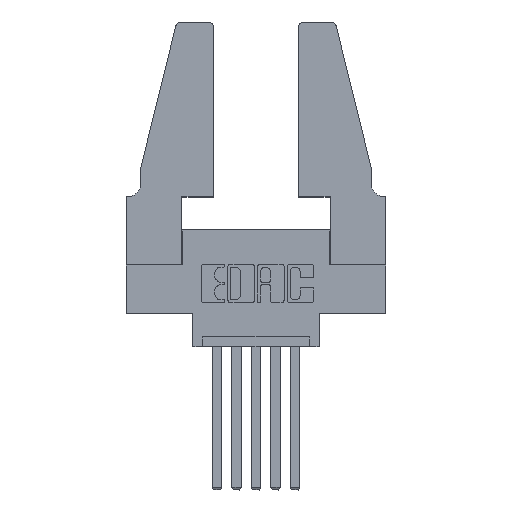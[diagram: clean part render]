
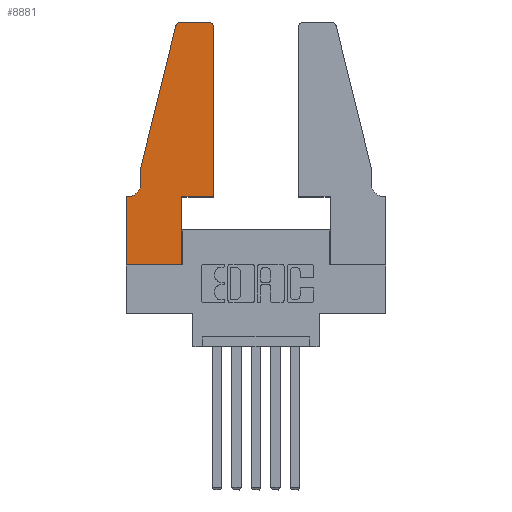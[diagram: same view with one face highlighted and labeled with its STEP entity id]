
A CAD part, top view. The second image highlights one B-rep face of the part: STEP entity #8881.
In plain terms, the highlighted planar face has unit normal (0, 0, 1).
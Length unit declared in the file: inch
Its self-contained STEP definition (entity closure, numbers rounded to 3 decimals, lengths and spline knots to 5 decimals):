
#51 = ORIENTED_EDGE ( 'NONE', *, *, #616, .T. ) ;
#91 = LINE ( 'NONE', #6774, #6468 ) ;
#209 = DIRECTION ( 'NONE',  ( 0., 0., 1. ) ) ;
#402 = AXIS2_PLACEMENT_3D ( 'NONE', #3626, #8668, #4568 ) ;
#415 = VERTEX_POINT ( 'NONE', #6234 ) ;
#616 = EDGE_CURVE ( 'NONE', #1237, #3128, #10781, .T. ) ;
#669 = ORIENTED_EDGE ( 'NONE', *, *, #1518, .T. ) ;
#771 = AXIS2_PLACEMENT_3D ( 'NONE', #8597, #209, #8660 ) ;
#1116 = ORIENTED_EDGE ( 'NONE', *, *, #4676, .T. ) ;
#1237 = VERTEX_POINT ( 'NONE', #10188 ) ;
#1250 = ORIENTED_EDGE ( 'NONE', *, *, #7082, .T. ) ;
#1518 = EDGE_CURVE ( 'NONE', #6402, #9654, #10625, .T. ) ;
#1603 = EDGE_CURVE ( 'NONE', #9789, #9514, #8399, .T. ) ;
#1641 = DIRECTION ( 'NONE',  ( 0., -1., 0. ) ) ;
#1747 = VECTOR ( 'NONE', #6673, 39.37008 ) ;
#1919 = PLANE ( 'NONE',  #771 ) ;
#2002 = LINE ( 'NONE', #3470, #1747 ) ;
#2590 = DIRECTION ( 'NONE',  ( 0., -1., 0. ) ) ;
#2674 = VERTEX_POINT ( 'NONE', #9841 ) ;
#2736 = CARTESIAN_POINT ( 'NONE',  ( 0., 0., 0.37 ) ) ;
#2806 = CARTESIAN_POINT ( 'NONE',  ( 0.0755, 0.42, 0.37 ) ) ;
#3128 = VERTEX_POINT ( 'NONE', #8133 ) ;
#3470 = CARTESIAN_POINT ( 'NONE',  ( 0.0755, 0.35, 0.37 ) ) ;
#3584 = DIRECTION ( 'NONE',  ( 1., 0., 0. ) ) ;
#3597 = CIRCLE ( 'NONE', #9255, 0.03 ) ;
#3626 = CARTESIAN_POINT ( 'NONE',  ( 0.0055, 0.42, 0.37 ) ) ;
#3688 = CARTESIAN_POINT ( 'NONE',  ( 0., 0.35, 0.37 ) ) ;
#3951 = DIRECTION ( 'NONE',  ( 0., 1., 0. ) ) ;
#4238 = CIRCLE ( 'NONE', #402, 0.07 ) ;
#4302 = EDGE_CURVE ( 'NONE', #9654, #9288, #3597, .T. ) ;
#4568 = DIRECTION ( 'NONE',  ( -1., 0., 0. ) ) ;
#4573 = DIRECTION ( 'NONE',  ( 1., 0., 0. ) ) ;
#4646 = LINE ( 'NONE', #8347, #8072 ) ;
#4676 = EDGE_CURVE ( 'NONE', #9514, #6031, #4238, .T. ) ;
#4728 = CARTESIAN_POINT ( 'NONE',  ( 0.2605, 1.25, 0.37 ) ) ;
#4741 = ORIENTED_EDGE ( 'NONE', *, *, #1603, .T. ) ;
#5018 = VERTEX_POINT ( 'NONE', #6386 ) ;
#5181 = ORIENTED_EDGE ( 'NONE', *, *, #5581, .T. ) ;
#5260 = LINE ( 'NONE', #2736, #5277 ) ;
#5277 = VECTOR ( 'NONE', #3584, 39.37008 ) ;
#5581 = EDGE_CURVE ( 'NONE', #2674, #1237, #8578, .T. ) ;
#5606 = CARTESIAN_POINT ( 'NONE',  ( 0.284, 1.22, 0.37 ) ) ;
#5708 = ORIENTED_EDGE ( 'NONE', *, *, #8925, .T. ) ;
#5906 = CARTESIAN_POINT ( 'NONE',  ( 0.25487, 1.22718, 0.37 ) ) ;
#6031 = VERTEX_POINT ( 'NONE', #8395 ) ;
#6033 = VECTOR ( 'NONE', #9230, 39.37008 ) ;
#6234 = CARTESIAN_POINT ( 'NONE',  ( 0., 0., 0.37 ) ) ;
#6386 = CARTESIAN_POINT ( 'NONE',  ( 0.2865, 0., 0.37 ) ) ;
#6402 = VERTEX_POINT ( 'NONE', #8605 ) ;
#6468 = VECTOR ( 'NONE', #2590, 39.37008 ) ;
#6477 = CARTESIAN_POINT ( 'NONE',  ( 0.0755, 0.5, 0.37 ) ) ;
#6502 = DIRECTION ( 'NONE',  ( -0.239, -0.971, 0. ) ) ;
#6504 = CARTESIAN_POINT ( 'NONE',  ( 0.4505, 0.35, 0.37 ) ) ;
#6572 = VECTOR ( 'NONE', #9714, 39.37008 ) ;
#6673 = DIRECTION ( 'NONE',  ( -1., 0., 0. ) ) ;
#6753 = ORIENTED_EDGE ( 'NONE', *, *, #9842, .T. ) ;
#6774 = CARTESIAN_POINT ( 'NONE',  ( 0., 0., 0.37 ) ) ;
#6972 = EDGE_CURVE ( 'NONE', #9288, #9789, #4646, .T. ) ;
#6982 = AXIS2_PLACEMENT_3D ( 'NONE', #7189, #9736, #4573 ) ;
#7082 = EDGE_CURVE ( 'NONE', #3128, #6402, #8204, .T. ) ;
#7117 = ORIENTED_EDGE ( 'NONE', *, *, #7146, .T. ) ;
#7146 = EDGE_CURVE ( 'NONE', #9051, #415, #91, .T. ) ;
#7189 = CARTESIAN_POINT ( 'NONE',  ( 0.4205, 1.22, 0.37 ) ) ;
#7245 = DIRECTION ( 'NONE',  ( 0., 0., 1. ) ) ;
#7310 = DIRECTION ( 'NONE',  ( -1., 0., 0. ) ) ;
#7571 = ORIENTED_EDGE ( 'NONE', *, *, #6972, .T. ) ;
#7639 = VECTOR ( 'NONE', #3951, 39.37008 ) ;
#7750 = VECTOR ( 'NONE', #1641, 39.37008 ) ;
#7915 = EDGE_LOOP ( 'NONE', ( #669, #9835, #7571, #4741, #1116, #7928, #7117, #5708, #6753, #5181, #51, #1250 ) ) ;
#7928 = ORIENTED_EDGE ( 'NONE', *, *, #9399, .T. ) ;
#8072 = VECTOR ( 'NONE', #6502, 39.37008 ) ;
#8133 = CARTESIAN_POINT ( 'NONE',  ( 0.4505, 1.22, 0.37 ) ) ;
#8204 = CIRCLE ( 'NONE', #6982, 0.03 ) ;
#8347 = CARTESIAN_POINT ( 'NONE',  ( 0.0755, 0.5, 0.37 ) ) ;
#8395 = CARTESIAN_POINT ( 'NONE',  ( 0.0055, 0.35, 0.37 ) ) ;
#8399 = LINE ( 'NONE', #6477, #7750 ) ;
#8578 = LINE ( 'NONE', #10343, #6572 ) ;
#8597 = CARTESIAN_POINT ( 'NONE',  ( 0., 0.35, 0.37 ) ) ;
#8605 = CARTESIAN_POINT ( 'NONE',  ( 0.4205, 1.25, 0.37 ) ) ;
#8660 = DIRECTION ( 'NONE',  ( 1., 0., 0. ) ) ;
#8668 = DIRECTION ( 'NONE',  ( 0., 0., -1. ) ) ;
#8881 = ADVANCED_FACE ( 'NONE', ( #9493 ), #1919, .T. ) ;
#8925 = EDGE_CURVE ( 'NONE', #415, #5018, #5260, .T. ) ;
#9011 = CARTESIAN_POINT ( 'NONE',  ( 0.0755, 0.5, 0.37 ) ) ;
#9048 = DIRECTION ( 'NONE',  ( 1., 0., 0. ) ) ;
#9051 = VERTEX_POINT ( 'NONE', #3688 ) ;
#9230 = DIRECTION ( 'NONE',  ( 0., 1., 0. ) ) ;
#9255 = AXIS2_PLACEMENT_3D ( 'NONE', #5606, #7245, #9048 ) ;
#9288 = VERTEX_POINT ( 'NONE', #5906 ) ;
#9332 = VECTOR ( 'NONE', #7310, 39.37008 ) ;
#9399 = EDGE_CURVE ( 'NONE', #6031, #9051, #2002, .T. ) ;
#9493 = FACE_OUTER_BOUND ( 'NONE', #7915, .T. ) ;
#9514 = VERTEX_POINT ( 'NONE', #2806 ) ;
#9608 = CARTESIAN_POINT ( 'NONE',  ( 0.284, 1.25, 0.37 ) ) ;
#9654 = VERTEX_POINT ( 'NONE', #9608 ) ;
#9714 = DIRECTION ( 'NONE',  ( 1., 0., 0. ) ) ;
#9736 = DIRECTION ( 'NONE',  ( 0., 0., 1. ) ) ;
#9789 = VERTEX_POINT ( 'NONE', #9011 ) ;
#9835 = ORIENTED_EDGE ( 'NONE', *, *, #4302, .T. ) ;
#9841 = CARTESIAN_POINT ( 'NONE',  ( 0.2865, 0.35, 0.37 ) ) ;
#9842 = EDGE_CURVE ( 'NONE', #5018, #2674, #10520, .T. ) ;
#10035 = CARTESIAN_POINT ( 'NONE',  ( 0.2865, 0.35, 0.37 ) ) ;
#10188 = CARTESIAN_POINT ( 'NONE',  ( 0.4505, 0.35, 0.37 ) ) ;
#10343 = CARTESIAN_POINT ( 'NONE',  ( 0.4505, 0.35, 0.37 ) ) ;
#10520 = LINE ( 'NONE', #10035, #6033 ) ;
#10625 = LINE ( 'NONE', #4728, #9332 ) ;
#10781 = LINE ( 'NONE', #6504, #7639 ) ;
